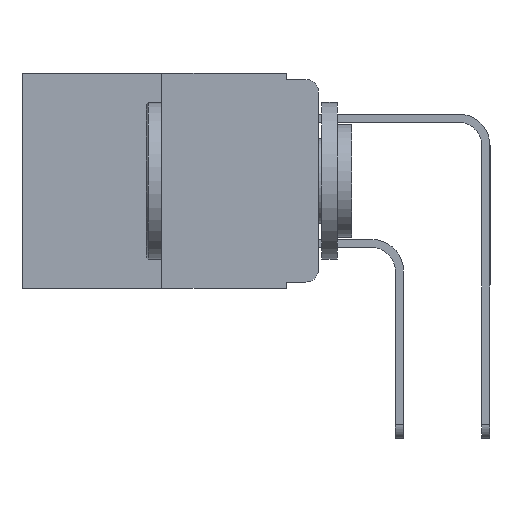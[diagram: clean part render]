
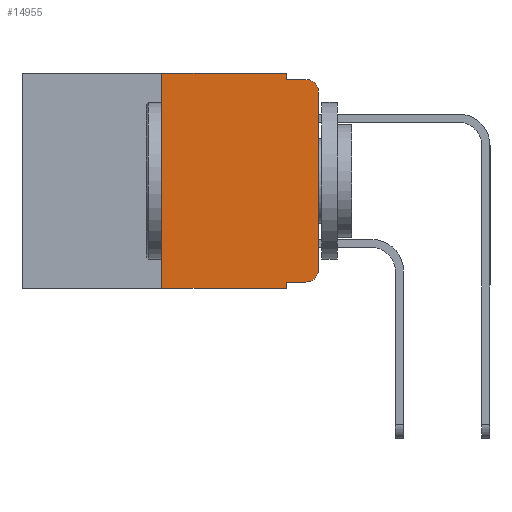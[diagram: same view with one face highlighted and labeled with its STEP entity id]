
A CAD part, left-side view. The second image highlights one B-rep face of the part: STEP entity #14955.
In plain terms, the highlighted planar face has unit normal (-1, 0, 0).
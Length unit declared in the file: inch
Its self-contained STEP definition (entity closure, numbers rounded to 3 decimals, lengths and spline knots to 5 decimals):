
#73 = VERTEX_POINT ( 'NONE', #8357 ) ;
#123 = CARTESIAN_POINT ( 'NONE',  ( 0., 0.051, -0.01 ) ) ;
#188 = VECTOR ( 'NONE', #191, 39.37008 ) ;
#191 = DIRECTION ( 'NONE',  ( 0., 0., -1. ) ) ;
#498 = VECTOR ( 'NONE', #11575, 39.37008 ) ;
#541 = CARTESIAN_POINT ( 'NONE',  ( 0., 0.051, -0.333 ) ) ;
#784 = CARTESIAN_POINT ( 'NONE',  ( 0., 0.051, -0.333 ) ) ;
#900 = EDGE_CURVE ( 'NONE', #11186, #73, #6890, .T. ) ;
#1230 = CIRCLE ( 'NONE', #10142, 0.02 ) ;
#1340 = CARTESIAN_POINT ( 'NONE',  ( 0., 0.25, 0. ) ) ;
#1594 = DIRECTION ( 'NONE',  ( 0., -1., 0. ) ) ;
#1596 = ORIENTED_EDGE ( 'NONE', *, *, #9831, .T. ) ;
#1783 = VECTOR ( 'NONE', #16215, 39.37008 ) ;
#2570 = VECTOR ( 'NONE', #8769, 39.37008 ) ;
#2669 = CARTESIAN_POINT ( 'NONE',  ( 0., 0.02, -0.313 ) ) ;
#2946 = PLANE ( 'NONE',  #10881 ) ;
#2956 = AXIS2_PLACEMENT_3D ( 'NONE', #2669, #12476, #4156 ) ;
#3458 = CARTESIAN_POINT ( 'NONE',  ( 0., 0.02, -0.03 ) ) ;
#4085 = VERTEX_POINT ( 'NONE', #1340 ) ;
#4156 = DIRECTION ( 'NONE',  ( 0., 0., -1. ) ) ;
#4412 = CARTESIAN_POINT ( 'NONE',  ( 0., 0.473, 0. ) ) ;
#4914 = DIRECTION ( 'NONE',  ( 0., 0., -1. ) ) ;
#5213 = EDGE_CURVE ( 'NONE', #9168, #11186, #9364, .T. ) ;
#5495 = ORIENTED_EDGE ( 'NONE', *, *, #900, .T. ) ;
#5602 = LINE ( 'NONE', #541, #8910 ) ;
#5800 = EDGE_LOOP ( 'NONE', ( #5495, #6396, #15741, #9459, #7496, #14701, #1596, #16796, #17216, #15150 ) ) ;
#5888 = DIRECTION ( 'NONE',  ( 0., 0., -1. ) ) ;
#5917 = CARTESIAN_POINT ( 'NONE',  ( 0., 0.25, 0. ) ) ;
#6197 = EDGE_CURVE ( 'NONE', #13456, #9168, #5602, .T. ) ;
#6290 = LINE ( 'NONE', #123, #16680 ) ;
#6396 = ORIENTED_EDGE ( 'NONE', *, *, #17989, .T. ) ;
#6415 = CARTESIAN_POINT ( 'NONE',  ( 0., 0.051, -0.343 ) ) ;
#6519 = LINE ( 'NONE', #5917, #13335 ) ;
#6585 = EDGE_CURVE ( 'NONE', #4085, #16599, #11443, .T. ) ;
#6890 = LINE ( 'NONE', #17644, #2570 ) ;
#7325 = DIRECTION ( 'NONE',  ( 0., 0., 1. ) ) ;
#7496 = ORIENTED_EDGE ( 'NONE', *, *, #6585, .F. ) ;
#7905 = LINE ( 'NONE', #14269, #188 ) ;
#8357 = CARTESIAN_POINT ( 'NONE',  ( 0., 0., -0.03 ) ) ;
#8769 = DIRECTION ( 'NONE',  ( 0., 0., 1. ) ) ;
#8910 = VECTOR ( 'NONE', #15880, 39.37008 ) ;
#9016 = EDGE_CURVE ( 'NONE', #13456, #13991, #7905, .T. ) ;
#9168 = VERTEX_POINT ( 'NONE', #17527 ) ;
#9364 = CIRCLE ( 'NONE', #2956, 0.02 ) ;
#9459 = ORIENTED_EDGE ( 'NONE', *, *, #13520, .F. ) ;
#9543 = CARTESIAN_POINT ( 'NONE',  ( 0., 0.051, 0. ) ) ;
#9553 = CARTESIAN_POINT ( 'NONE',  ( 0., 0.473, -0.343 ) ) ;
#9609 = DIRECTION ( 'NONE',  ( 0., 0., -1. ) ) ;
#9819 = CARTESIAN_POINT ( 'NONE',  ( 0., 0.051, -0.01 ) ) ;
#9831 = EDGE_CURVE ( 'NONE', #17667, #13991, #12592, .T. ) ;
#10142 = AXIS2_PLACEMENT_3D ( 'NONE', #3458, #13194, #4914 ) ;
#10278 = CARTESIAN_POINT ( 'NONE',  ( 0., 0.473, 0. ) ) ;
#10881 = AXIS2_PLACEMENT_3D ( 'NONE', #4412, #14065, #5888 ) ;
#11153 = CARTESIAN_POINT ( 'NONE',  ( 0., 0.051, 0. ) ) ;
#11186 = VERTEX_POINT ( 'NONE', #16151 ) ;
#11443 = LINE ( 'NONE', #10278, #498 ) ;
#11528 = CARTESIAN_POINT ( 'NONE',  ( 0., 0.02, -0.01 ) ) ;
#11575 = DIRECTION ( 'NONE',  ( 0., -1., 0. ) ) ;
#11690 = VERTEX_POINT ( 'NONE', #9819 ) ;
#11749 = EDGE_CURVE ( 'NONE', #17667, #4085, #6519, .T. ) ;
#12476 = DIRECTION ( 'NONE',  ( -1., 0., 0. ) ) ;
#12592 = LINE ( 'NONE', #9553, #1783 ) ;
#13194 = DIRECTION ( 'NONE',  ( -1., 0., 0. ) ) ;
#13335 = VECTOR ( 'NONE', #7325, 39.37008 ) ;
#13456 = VERTEX_POINT ( 'NONE', #784 ) ;
#13520 = EDGE_CURVE ( 'NONE', #16599, #11690, #17552, .T. ) ;
#13991 = VERTEX_POINT ( 'NONE', #6415 ) ;
#14007 = VECTOR ( 'NONE', #9609, 39.37008 ) ;
#14065 = DIRECTION ( 'NONE',  ( 1., 0., 0. ) ) ;
#14269 = CARTESIAN_POINT ( 'NONE',  ( 0., 0.051, 0. ) ) ;
#14415 = EDGE_CURVE ( 'NONE', #11690, #17844, #6290, .T. ) ;
#14567 = FACE_OUTER_BOUND ( 'NONE', #5800, .T. ) ;
#14701 = ORIENTED_EDGE ( 'NONE', *, *, #11749, .F. ) ;
#14955 = ADVANCED_FACE ( 'NONE', ( #14567 ), #2946, .F. ) ;
#15082 = CARTESIAN_POINT ( 'NONE',  ( 0., 0.25, -0.343 ) ) ;
#15150 = ORIENTED_EDGE ( 'NONE', *, *, #5213, .T. ) ;
#15741 = ORIENTED_EDGE ( 'NONE', *, *, #14415, .F. ) ;
#15880 = DIRECTION ( 'NONE',  ( 0., -1., 0. ) ) ;
#16151 = CARTESIAN_POINT ( 'NONE',  ( 0., 0., -0.313 ) ) ;
#16215 = DIRECTION ( 'NONE',  ( 0., -1., 0. ) ) ;
#16599 = VERTEX_POINT ( 'NONE', #11153 ) ;
#16680 = VECTOR ( 'NONE', #1594, 39.37008 ) ;
#16796 = ORIENTED_EDGE ( 'NONE', *, *, #9016, .F. ) ;
#17216 = ORIENTED_EDGE ( 'NONE', *, *, #6197, .T. ) ;
#17527 = CARTESIAN_POINT ( 'NONE',  ( 0., 0.02, -0.333 ) ) ;
#17552 = LINE ( 'NONE', #9543, #14007 ) ;
#17644 = CARTESIAN_POINT ( 'NONE',  ( 0., 0., 0. ) ) ;
#17667 = VERTEX_POINT ( 'NONE', #15082 ) ;
#17844 = VERTEX_POINT ( 'NONE', #11528 ) ;
#17989 = EDGE_CURVE ( 'NONE', #73, #17844, #1230, .T. ) ;
